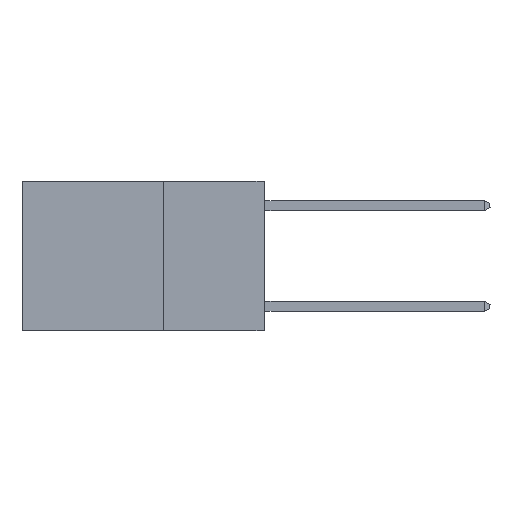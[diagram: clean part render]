
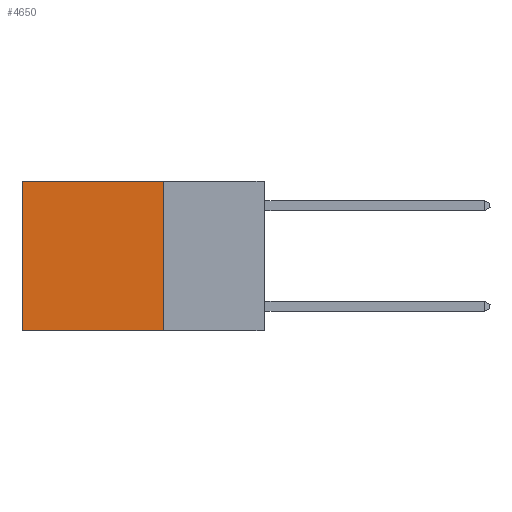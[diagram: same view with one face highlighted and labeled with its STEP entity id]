
A CAD part, left-side view. The second image highlights one B-rep face of the part: STEP entity #4650.
In plain terms, the highlighted planar face has unit normal (-1, 0, 0).
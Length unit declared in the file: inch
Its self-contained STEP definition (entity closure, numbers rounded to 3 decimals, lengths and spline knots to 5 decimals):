
#345 = ORIENTED_EDGE ( 'NONE', *, *, #6457, .F. ) ;
#972 = DIRECTION ( 'NONE',  ( 0., 1., 0. ) ) ;
#1074 = AXIS2_PLACEMENT_3D ( 'NONE', #16486, #9663, #15081 ) ;
#1227 = ORIENTED_EDGE ( 'NONE', *, *, #4367, .T. ) ;
#1376 = LINE ( 'NONE', #7012, #14881 ) ;
#1504 = DIRECTION ( 'NONE',  ( 0., 1., 0. ) ) ;
#1985 = CARTESIAN_POINT ( 'NONE',  ( 0.2625, 0.6, -0.37 ) ) ;
#2904 = CARTESIAN_POINT ( 'NONE',  ( 0.2625, 0.25, 0. ) ) ;
#3778 = FACE_OUTER_BOUND ( 'NONE', #10803, .T. ) ;
#3868 = VECTOR ( 'NONE', #972, 39.37008 ) ;
#4025 = ORIENTED_EDGE ( 'NONE', *, *, #4544, .F. ) ;
#4367 = EDGE_CURVE ( 'NONE', #13910, #14746, #16158, .T. ) ;
#4462 = PLANE ( 'NONE',  #1074 ) ;
#4544 = EDGE_CURVE ( 'NONE', #13910, #13278, #7769, .T. ) ;
#4650 = ADVANCED_FACE ( 'NONE', ( #3778 ), #4462, .F. ) ;
#5544 = CARTESIAN_POINT ( 'NONE',  ( 0.2625, 0.25, -0.37 ) ) ;
#6267 = CARTESIAN_POINT ( 'NONE',  ( 0.2625, 0.25, 0. ) ) ;
#6457 = EDGE_CURVE ( 'NONE', #13278, #9767, #12400, .T. ) ;
#7012 = CARTESIAN_POINT ( 'NONE',  ( 0.2625, 0.6, 0. ) ) ;
#7769 = LINE ( 'NONE', #14412, #10543 ) ;
#8698 = CARTESIAN_POINT ( 'NONE',  ( 0.2625, 0.6, 0. ) ) ;
#9421 = CARTESIAN_POINT ( 'NONE',  ( 0.2625, 0.25, -0.37 ) ) ;
#9663 = DIRECTION ( 'NONE',  ( 1., 0., 0. ) ) ;
#9767 = VERTEX_POINT ( 'NONE', #1985 ) ;
#10543 = VECTOR ( 'NONE', #13295, 39.37008 ) ;
#10803 = EDGE_LOOP ( 'NONE', ( #10849, #345, #4025, #1227 ) ) ;
#10849 = ORIENTED_EDGE ( 'NONE', *, *, #16810, .T. ) ;
#11054 = VECTOR ( 'NONE', #1504, 39.37008 ) ;
#12400 = LINE ( 'NONE', #5544, #11054 ) ;
#13278 = VERTEX_POINT ( 'NONE', #9421 ) ;
#13295 = DIRECTION ( 'NONE',  ( 0., 0., -1. ) ) ;
#13597 = DIRECTION ( 'NONE',  ( 0., 0., -1. ) ) ;
#13910 = VERTEX_POINT ( 'NONE', #6267 ) ;
#14412 = CARTESIAN_POINT ( 'NONE',  ( 0.2625, 0.25, 0. ) ) ;
#14746 = VERTEX_POINT ( 'NONE', #8698 ) ;
#14881 = VECTOR ( 'NONE', #13597, 39.37008 ) ;
#15081 = DIRECTION ( 'NONE',  ( 0., 0., -1. ) ) ;
#16158 = LINE ( 'NONE', #2904, #3868 ) ;
#16486 = CARTESIAN_POINT ( 'NONE',  ( 0.2625, 0.25, 0. ) ) ;
#16810 = EDGE_CURVE ( 'NONE', #14746, #9767, #1376, .T. ) ;
